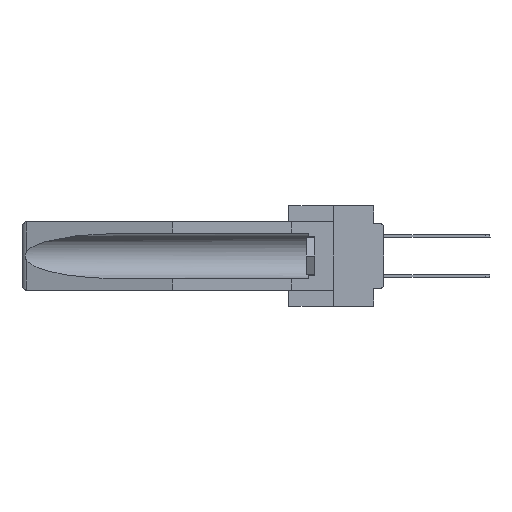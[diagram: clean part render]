
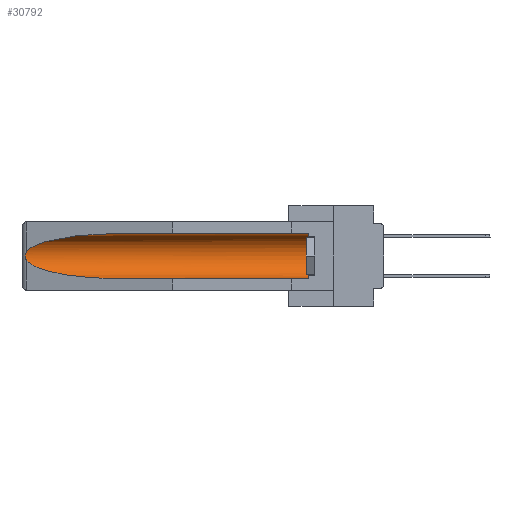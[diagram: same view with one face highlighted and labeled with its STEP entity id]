
A CAD part, left-side view. The second image highlights one B-rep face of the part: STEP entity #30792.
In plain terms, the highlighted cylindrical face has radius 2.857 mm (diameter 5.715 mm), a partial arc.
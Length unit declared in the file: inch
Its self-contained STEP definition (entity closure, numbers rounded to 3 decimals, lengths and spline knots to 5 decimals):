
#236 = EDGE_CURVE ( 'NONE', #34589, #16743, #24500, .T. ) ;
#1376 = VERTEX_POINT ( 'NONE', #17624 ) ;
#2332 = DIRECTION ( 'NONE',  ( 0., 0., 1. ) ) ;
#2863 = CARTESIAN_POINT ( 'NONE',  ( 0.155, 0.126, -0.1715 ) ) ;
#5089 = CARTESIAN_POINT ( 'NONE',  ( 0.26537, 1.52718, -0.14972 ) ) ;
#5259 = CARTESIAN_POINT ( 'NONE',  ( 0.155, -0.30754, -0.1715 ) ) ;
#6682 =( BOUNDED_CURVE ( )  B_SPLINE_CURVE ( 3, ( #10566, #21366, #7649, #16273 ),
 .UNSPECIFIED., .F., .F. ) 
 B_SPLINE_CURVE_WITH_KNOTS ( ( 4, 4 ),
 ( 0.1948, 1.5708 ),
 .UNSPECIFIED. ) 
 CURVE ( )  GEOMETRIC_REPRESENTATION_ITEM ( )  RATIONAL_B_SPLINE_CURVE ( ( 1., 0.848, 0.848, 1. ) ) 
 REPRESENTATION_ITEM ( '' )  );
#6969 = VERTEX_POINT ( 'NONE', #35546 ) ;
#7649 = CARTESIAN_POINT ( 'NONE',  ( 0.21114, 1.30732, -0.284 ) ) ;
#7775 = DIRECTION ( 'NONE',  ( 0., 1., 0. ) ) ;
#7872 = CARTESIAN_POINT ( 'NONE',  ( 0.2675, 1.53308, -0.17534 ) ) ;
#8076 = CYLINDRICAL_SURFACE ( 'NONE', #13003, 0.1125 ) ;
#8337 = CARTESIAN_POINT ( 'NONE',  ( 0.2675, 1.53308, -0.16763 ) ) ;
#8369 = LINE ( 'NONE', #9938, #10551 ) ;
#9938 = CARTESIAN_POINT ( 'NONE',  ( 0.155, -0.30754, -0.059 ) ) ;
#10551 = VECTOR ( 'NONE', #7775, 39.37008 ) ;
#10566 = CARTESIAN_POINT ( 'NONE',  ( 0.26537, 1.52718, -0.19328 ) ) ;
#10785 = CARTESIAN_POINT ( 'NONE',  ( 0.26537, 1.52718, -0.19328 ) ) ;
#12030 = CIRCLE ( 'NONE', #24612, 0.1125 ) ;
#12569 = CARTESIAN_POINT ( 'NONE',  ( 0.26537, 1.52718, -0.14972 ) ) ;
#12743 = CARTESIAN_POINT ( 'NONE',  ( 0.155, 1.07973, -0.059 ) ) ;
#13003 = AXIS2_PLACEMENT_3D ( 'NONE', #5259, #33265, #2332 ) ;
#13028 = CARTESIAN_POINT ( 'NONE',  ( 0.155, 0.126, -0.284 ) ) ;
#13577 = CARTESIAN_POINT ( 'NONE',  ( 0.26654, 1.53092, -0.15636 ) ) ;
#13608 = CARTESIAN_POINT ( 'NONE',  ( 0.155, -0.30754, -0.284 ) ) ;
#13611 =( BOUNDED_CURVE ( )  B_SPLINE_CURVE ( 3, ( #28956, #23605, #17792, #12569 ),
 .UNSPECIFIED., .F., .F. ) 
 B_SPLINE_CURVE_WITH_KNOTS ( ( 4, 4 ),
 ( 4.71239, 6.08839 ),
 .UNSPECIFIED. ) 
 CURVE ( )  GEOMETRIC_REPRESENTATION_ITEM ( )  RATIONAL_B_SPLINE_CURVE ( ( 1., 0.848, 0.848, 1. ) ) 
 REPRESENTATION_ITEM ( '' )  );
#13816 = CARTESIAN_POINT ( 'NONE',  ( 0.26597, 1.5296, -0.19026 ) ) ;
#13861 = CARTESIAN_POINT ( 'NONE',  ( 0.26537, 1.52718, -0.14972 ) ) ;
#13938 = CARTESIAN_POINT ( 'NONE',  ( 0.2673, 1.5327, -0.16383 ) ) ;
#14437 = ORIENTED_EDGE ( 'NONE', *, *, #28336, .T. ) ;
#14748 = ORIENTED_EDGE ( 'NONE', *, *, #33632, .T. ) ;
#16092 = VERTEX_POINT ( 'NONE', #12743 ) ;
#16273 = CARTESIAN_POINT ( 'NONE',  ( 0.155, 1.07973, -0.284 ) ) ;
#16498 = CARTESIAN_POINT ( 'NONE',  ( 0.26655, 1.53094, -0.18657 ) ) ;
#16743 = VERTEX_POINT ( 'NONE', #25862 ) ;
#17624 = CARTESIAN_POINT ( 'NONE',  ( 0.155, 1.07973, -0.284 ) ) ;
#17792 = CARTESIAN_POINT ( 'NONE',  ( 0.25451, 1.48313, -0.09465 ) ) ;
#19542 = ORIENTED_EDGE ( 'NONE', *, *, #236, .T. ) ;
#20456 = EDGE_CURVE ( 'NONE', #25572, #1376, #23707, .T. ) ;
#21366 = CARTESIAN_POINT ( 'NONE',  ( 0.25451, 1.48313, -0.24835 ) ) ;
#22407 = VECTOR ( 'NONE', #33013, 39.37008 ) ;
#22495 = ORIENTED_EDGE ( 'NONE', *, *, #20456, .F. ) ;
#22687 = ORIENTED_EDGE ( 'NONE', *, *, #32562, .T. ) ;
#23605 = CARTESIAN_POINT ( 'NONE',  ( 0.21114, 1.30732, -0.059 ) ) ;
#23707 = LINE ( 'NONE', #13608, #22407 ) ;
#24163 = EDGE_LOOP ( 'NONE', ( #14748, #19542, #32332, #22495, #14437, #22687 ) ) ;
#24500 = B_SPLINE_CURVE_WITH_KNOTS ( 'NONE', 3,
 ( #5089, #30555, #13577, #13938, #8337, #7872, #30435, #16498, #13816, #10785 ),
 .UNSPECIFIED., .F., .F.,
 ( 4, 2, 2, 2, 4 ),
 ( 0., 0.00029, 0.00058, 0.00087, 0.00117 ),
 .UNSPECIFIED. ) ;
#24612 = AXIS2_PLACEMENT_3D ( 'NONE', #2863, #30311, #31989 ) ;
#25572 = VERTEX_POINT ( 'NONE', #13028 ) ;
#25862 = CARTESIAN_POINT ( 'NONE',  ( 0.26537, 1.52718, -0.19328 ) ) ;
#28336 = EDGE_CURVE ( 'NONE', #25572, #6969, #12030, .T. ) ;
#28468 = FACE_OUTER_BOUND ( 'NONE', #24163, .T. ) ;
#28956 = CARTESIAN_POINT ( 'NONE',  ( 0.155, 1.07973, -0.059 ) ) ;
#30311 = DIRECTION ( 'NONE',  ( 0., -1., 0. ) ) ;
#30435 = CARTESIAN_POINT ( 'NONE',  ( 0.2673, 1.53269, -0.17917 ) ) ;
#30555 = CARTESIAN_POINT ( 'NONE',  ( 0.26597, 1.52961, -0.15275 ) ) ;
#30792 = ADVANCED_FACE ( 'NONE', ( #28468 ), #8076, .F. ) ;
#30944 = EDGE_CURVE ( 'NONE', #16743, #1376, #6682, .T. ) ;
#31989 = DIRECTION ( 'NONE',  ( 0., 0., 1. ) ) ;
#32332 = ORIENTED_EDGE ( 'NONE', *, *, #30944, .T. ) ;
#32562 = EDGE_CURVE ( 'NONE', #6969, #16092, #8369, .T. ) ;
#33013 = DIRECTION ( 'NONE',  ( 0., 1., 0. ) ) ;
#33265 = DIRECTION ( 'NONE',  ( 0., 1., 0. ) ) ;
#33632 = EDGE_CURVE ( 'NONE', #16092, #34589, #13611, .T. ) ;
#34589 = VERTEX_POINT ( 'NONE', #13861 ) ;
#35546 = CARTESIAN_POINT ( 'NONE',  ( 0.155, 0.126, -0.059 ) ) ;
